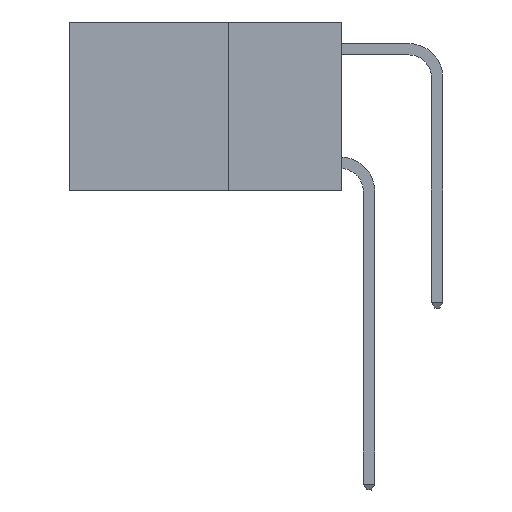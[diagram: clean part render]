
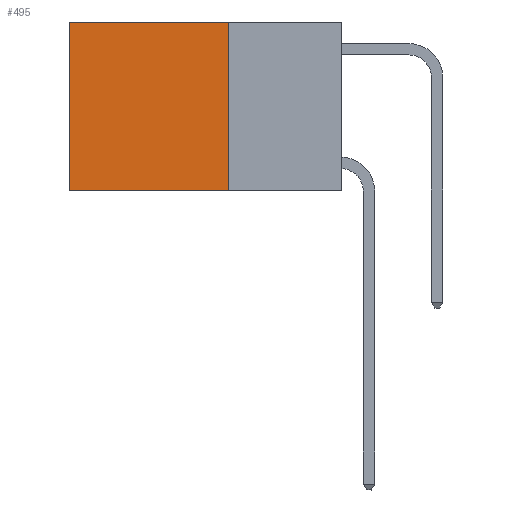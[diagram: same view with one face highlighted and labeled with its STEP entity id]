
A CAD part, left-side view. The second image highlights one B-rep face of the part: STEP entity #495.
In plain terms, the highlighted planar face has unit normal (-1, 0, 0).
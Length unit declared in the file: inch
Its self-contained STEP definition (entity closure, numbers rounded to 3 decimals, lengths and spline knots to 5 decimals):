
#106 = VECTOR ( 'NONE', #2253, 39.37008 ) ;
#140 = CARTESIAN_POINT ( 'NONE',  ( 0.2625, 0.6, 0. ) ) ;
#495 = ADVANCED_FACE ( 'NONE', ( #12328 ), #2646, .F. ) ;
#790 = EDGE_CURVE ( 'NONE', #10912, #1274, #8357, .T. ) ;
#850 = ORIENTED_EDGE ( 'NONE', *, *, #790, .T. ) ;
#1274 = VERTEX_POINT ( 'NONE', #8104 ) ;
#1357 = AXIS2_PLACEMENT_3D ( 'NONE', #6118, #8514, #3914 ) ;
#1942 = EDGE_LOOP ( 'NONE', ( #8618, #7059, #6018, #850 ) ) ;
#2166 = CARTESIAN_POINT ( 'NONE',  ( 0.2625, 0.25, 0. ) ) ;
#2253 = DIRECTION ( 'NONE',  ( 0., 1., 0. ) ) ;
#2646 = PLANE ( 'NONE',  #1357 ) ;
#3115 = CARTESIAN_POINT ( 'NONE',  ( 0.2625, 0.6, -0.37 ) ) ;
#3223 = VECTOR ( 'NONE', #10034, 39.37008 ) ;
#3777 = EDGE_CURVE ( 'NONE', #15103, #15085, #14762, .T. ) ;
#3886 = EDGE_CURVE ( 'NONE', #10912, #15103, #13745, .T. ) ;
#3914 = DIRECTION ( 'NONE',  ( 0., 0., -1. ) ) ;
#4885 = LINE ( 'NONE', #140, #8751 ) ;
#5020 = DIRECTION ( 'NONE',  ( 0., 1., 0. ) ) ;
#6008 = CARTESIAN_POINT ( 'NONE',  ( 0.2625, 0.25, 0. ) ) ;
#6018 = ORIENTED_EDGE ( 'NONE', *, *, #3886, .F. ) ;
#6118 = CARTESIAN_POINT ( 'NONE',  ( 0.2625, 0.25, 0. ) ) ;
#7059 = ORIENTED_EDGE ( 'NONE', *, *, #3777, .F. ) ;
#8104 = CARTESIAN_POINT ( 'NONE',  ( 0.2625, 0.6, 0. ) ) ;
#8357 = LINE ( 'NONE', #2166, #106 ) ;
#8435 = CARTESIAN_POINT ( 'NONE',  ( 0.2625, 0.25, -0.37 ) ) ;
#8514 = DIRECTION ( 'NONE',  ( 1., 0., 0. ) ) ;
#8618 = ORIENTED_EDGE ( 'NONE', *, *, #15627, .T. ) ;
#8751 = VECTOR ( 'NONE', #13313, 39.37008 ) ;
#10034 = DIRECTION ( 'NONE',  ( 0., 0., -1. ) ) ;
#10833 = VECTOR ( 'NONE', #5020, 39.37008 ) ;
#10912 = VERTEX_POINT ( 'NONE', #6008 ) ;
#11622 = CARTESIAN_POINT ( 'NONE',  ( 0.2625, 0.25, -0.37 ) ) ;
#12328 = FACE_OUTER_BOUND ( 'NONE', #1942, .T. ) ;
#12480 = CARTESIAN_POINT ( 'NONE',  ( 0.2625, 0.25, 0. ) ) ;
#13313 = DIRECTION ( 'NONE',  ( 0., 0., -1. ) ) ;
#13745 = LINE ( 'NONE', #12480, #3223 ) ;
#14762 = LINE ( 'NONE', #8435, #10833 ) ;
#15085 = VERTEX_POINT ( 'NONE', #3115 ) ;
#15103 = VERTEX_POINT ( 'NONE', #11622 ) ;
#15627 = EDGE_CURVE ( 'NONE', #1274, #15085, #4885, .T. ) ;
